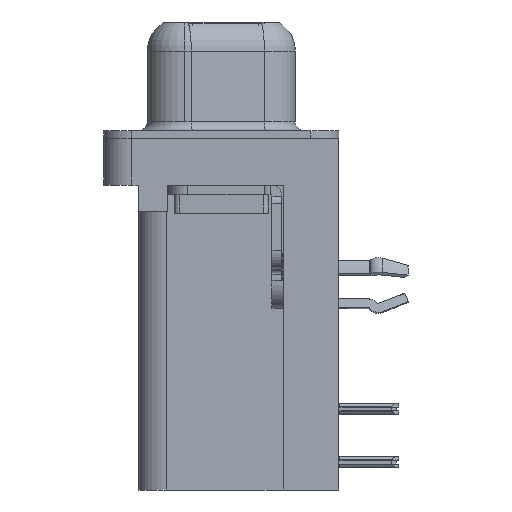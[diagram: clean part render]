
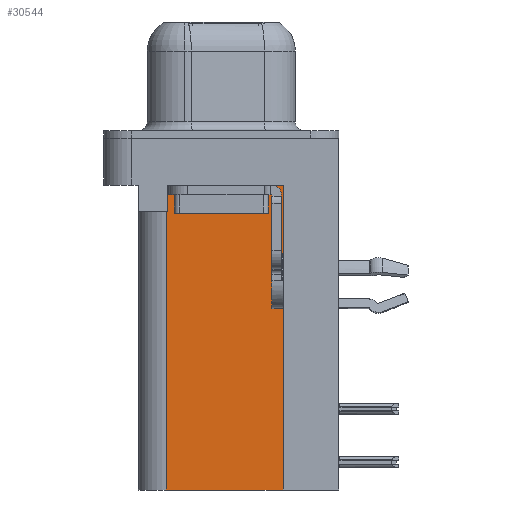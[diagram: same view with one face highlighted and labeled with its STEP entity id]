
A CAD part, left-side view. The second image highlights one B-rep face of the part: STEP entity #30544.
In plain terms, the highlighted planar face has unit normal (-1, 0, 0).
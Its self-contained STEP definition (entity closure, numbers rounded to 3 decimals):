
#181 = EDGE_CURVE ( 'NONE', #31630, #23054, #17972, .T. ) ;
#941 = CARTESIAN_POINT ( 'NONE',  ( 3.7, -3.295, -18.76 ) ) ;
#1512 = EDGE_CURVE ( 'NONE', #11080, #29208, #12137, .T. ) ;
#2352 = CARTESIAN_POINT ( 'NONE',  ( 3.7, 2.895, -3.9 ) ) ;
#3445 = PLANE ( 'NONE',  #29621 ) ;
#4183 = ORIENTED_EDGE ( 'NONE', *, *, #28384, .F. ) ;
#4794 = DIRECTION ( 'NONE',  ( 0., 1., 0. ) ) ;
#4900 = VERTEX_POINT ( 'NONE', #27032 ) ;
#5527 = CARTESIAN_POINT ( 'NONE',  ( 3.7, 2.925, -18.76 ) ) ;
#6218 = DIRECTION ( 'NONE',  ( 0., 0., 1. ) ) ;
#7302 = CARTESIAN_POINT ( 'NONE',  ( 3.7, 2.925, -18.76 ) ) ;
#7635 = VECTOR ( 'NONE', #24751, 1000. ) ;
#8191 = LINE ( 'NONE', #11184, #21594 ) ;
#8653 = LINE ( 'NONE', #25644, #14572 ) ;
#10119 = ORIENTED_EDGE ( 'NONE', *, *, #181, .F. ) ;
#10293 = CARTESIAN_POINT ( 'NONE',  ( 3.7, 2.925, -3.9 ) ) ;
#10679 = CARTESIAN_POINT ( 'NONE',  ( 3.7, 2.895, -2.5 ) ) ;
#11080 = VERTEX_POINT ( 'NONE', #24748 ) ;
#11184 = CARTESIAN_POINT ( 'NONE',  ( 3.7, -3.295, -18.76 ) ) ;
#12137 = LINE ( 'NONE', #22351, #12328 ) ;
#12328 = VECTOR ( 'NONE', #4794, 1000. ) ;
#12689 = LINE ( 'NONE', #20721, #27353 ) ;
#13500 = EDGE_CURVE ( 'NONE', #30283, #23054, #12689, .T. ) ;
#14572 = VECTOR ( 'NONE', #15656, 1000. ) ;
#15656 = DIRECTION ( 'NONE',  ( 0., 0., 1. ) ) ;
#17218 = EDGE_LOOP ( 'NONE', ( #22768, #32227, #29368, #10119, #4183, #28027 ) ) ;
#17885 = VECTOR ( 'NONE', #6218, 1000. ) ;
#17972 = LINE ( 'NONE', #7302, #17885 ) ;
#18178 = DIRECTION ( 'NONE',  ( 0., 1., 0. ) ) ;
#20721 = CARTESIAN_POINT ( 'NONE',  ( 3.7, 0., -3.9 ) ) ;
#21020 = DIRECTION ( 'NONE',  ( 0., 1., 0. ) ) ;
#21594 = VECTOR ( 'NONE', #28758, 1000. ) ;
#21922 = FACE_OUTER_BOUND ( 'NONE', #17218, .T. ) ;
#22351 = CARTESIAN_POINT ( 'NONE',  ( 3.7, -3.295, -2.5 ) ) ;
#22768 = ORIENTED_EDGE ( 'NONE', *, *, #1512, .T. ) ;
#22930 = EDGE_CURVE ( 'NONE', #29208, #30283, #26929, .T. ) ;
#23054 = VERTEX_POINT ( 'NONE', #10293 ) ;
#24748 = CARTESIAN_POINT ( 'NONE',  ( 3.7, -3.295, -2.5 ) ) ;
#24751 = DIRECTION ( 'NONE',  ( 0., 0., -1. ) ) ;
#25644 = CARTESIAN_POINT ( 'NONE',  ( 3.7, -3.295, -18.76 ) ) ;
#26699 = EDGE_CURVE ( 'NONE', #4900, #11080, #8653, .T. ) ;
#26929 = LINE ( 'NONE', #29846, #7635 ) ;
#27032 = CARTESIAN_POINT ( 'NONE',  ( 3.7, -3.295, -18.76 ) ) ;
#27353 = VECTOR ( 'NONE', #18178, 1000. ) ;
#28027 = ORIENTED_EDGE ( 'NONE', *, *, #26699, .T. ) ;
#28384 = EDGE_CURVE ( 'NONE', #4900, #31630, #8191, .T. ) ;
#28391 = DIRECTION ( 'NONE',  ( 1., 0., 0. ) ) ;
#28758 = DIRECTION ( 'NONE',  ( 0., 1., 0. ) ) ;
#29208 = VERTEX_POINT ( 'NONE', #10679 ) ;
#29368 = ORIENTED_EDGE ( 'NONE', *, *, #13500, .T. ) ;
#29621 = AXIS2_PLACEMENT_3D ( 'NONE', #941, #28391, #21020 ) ;
#29846 = CARTESIAN_POINT ( 'NONE',  ( 3.7, 2.895, -3.9 ) ) ;
#30283 = VERTEX_POINT ( 'NONE', #2352 ) ;
#30544 = ADVANCED_FACE ( 'NONE', ( #21922 ), #3445, .F. ) ;
#31630 = VERTEX_POINT ( 'NONE', #5527 ) ;
#32227 = ORIENTED_EDGE ( 'NONE', *, *, #22930, .T. ) ;
